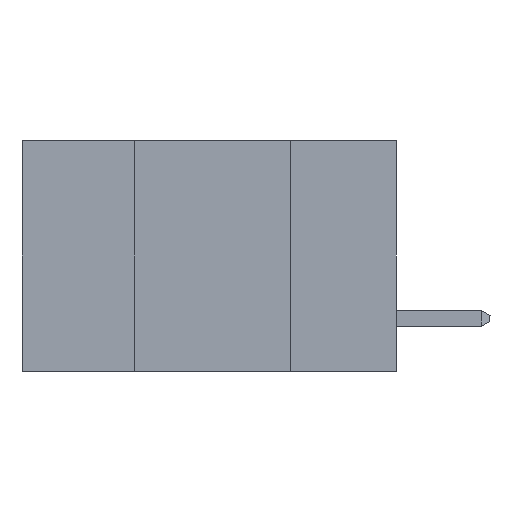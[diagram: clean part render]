
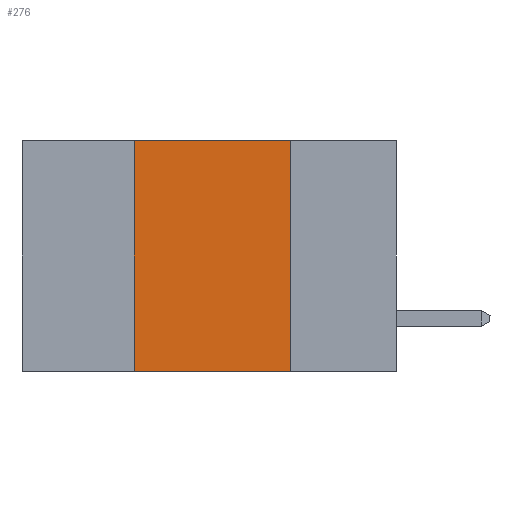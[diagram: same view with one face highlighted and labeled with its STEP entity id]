
A CAD part, left-side view. The second image highlights one B-rep face of the part: STEP entity #276.
In plain terms, the highlighted planar face has unit normal (-1, 0, 0).
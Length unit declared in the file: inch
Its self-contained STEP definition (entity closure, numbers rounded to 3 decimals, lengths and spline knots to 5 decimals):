
#276 = ADVANCED_FACE ( 'NONE', ( #9184 ), #2052, .F. ) ;
#1999 = CARTESIAN_POINT ( 'NONE',  ( 0., 0.17, -0.37 ) ) ;
#2052 = PLANE ( 'NONE',  #4214 ) ;
#2189 = VERTEX_POINT ( 'NONE', #4882 ) ;
#2202 = VERTEX_POINT ( 'NONE', #13288 ) ;
#2232 = EDGE_LOOP ( 'NONE', ( #3394, #4404, #9528, #5316 ) ) ;
#2272 = LINE ( 'NONE', #8390, #2754 ) ;
#2754 = VECTOR ( 'NONE', #10477, 39.37008 ) ;
#3055 = EDGE_CURVE ( 'NONE', #13031, #2189, #11218, .T. ) ;
#3204 = DIRECTION ( 'NONE',  ( 0., 0., -1. ) ) ;
#3394 = ORIENTED_EDGE ( 'NONE', *, *, #3055, .F. ) ;
#3498 = CARTESIAN_POINT ( 'NONE',  ( 0., 0.6, -0.37 ) ) ;
#3779 = VECTOR ( 'NONE', #7188, 39.37008 ) ;
#4214 = AXIS2_PLACEMENT_3D ( 'NONE', #6153, #8174, #3204 ) ;
#4404 = ORIENTED_EDGE ( 'NONE', *, *, #5187, .F. ) ;
#4781 = CARTESIAN_POINT ( 'NONE',  ( 0., 0.17, 0. ) ) ;
#4882 = CARTESIAN_POINT ( 'NONE',  ( 0., 0.17, -0.37 ) ) ;
#5101 = VECTOR ( 'NONE', #6523, 39.37008 ) ;
#5187 = EDGE_CURVE ( 'NONE', #13134, #13031, #10386, .T. ) ;
#5316 = ORIENTED_EDGE ( 'NONE', *, *, #6617, .T. ) ;
#5335 = CARTESIAN_POINT ( 'NONE',  ( 0., 0.6, 0. ) ) ;
#6050 = CARTESIAN_POINT ( 'NONE',  ( 0., 0.42, 0. ) ) ;
#6153 = CARTESIAN_POINT ( 'NONE',  ( 0., 0.6, 0. ) ) ;
#6523 = DIRECTION ( 'NONE',  ( 0., -1., 0. ) ) ;
#6617 = EDGE_CURVE ( 'NONE', #2202, #2189, #7664, .T. ) ;
#6772 = EDGE_CURVE ( 'NONE', #2202, #13134, #2272, .T. ) ;
#7188 = DIRECTION ( 'NONE',  ( 0., 0., -1. ) ) ;
#7664 = LINE ( 'NONE', #3498, #5101 ) ;
#8174 = DIRECTION ( 'NONE',  ( 1., 0., 0. ) ) ;
#8390 = CARTESIAN_POINT ( 'NONE',  ( 0., 0.42, -0.37 ) ) ;
#9184 = FACE_OUTER_BOUND ( 'NONE', #2232, .T. ) ;
#9528 = ORIENTED_EDGE ( 'NONE', *, *, #6772, .F. ) ;
#10386 = LINE ( 'NONE', #5335, #12176 ) ;
#10477 = DIRECTION ( 'NONE',  ( 0., 0., 1. ) ) ;
#11218 = LINE ( 'NONE', #1999, #3779 ) ;
#12176 = VECTOR ( 'NONE', #12478, 39.37008 ) ;
#12478 = DIRECTION ( 'NONE',  ( 0., -1., 0. ) ) ;
#13031 = VERTEX_POINT ( 'NONE', #4781 ) ;
#13134 = VERTEX_POINT ( 'NONE', #6050 ) ;
#13288 = CARTESIAN_POINT ( 'NONE',  ( 0., 0.42, -0.37 ) ) ;
